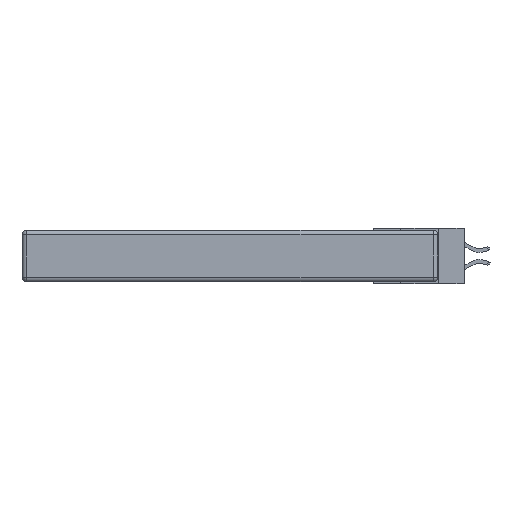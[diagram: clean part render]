
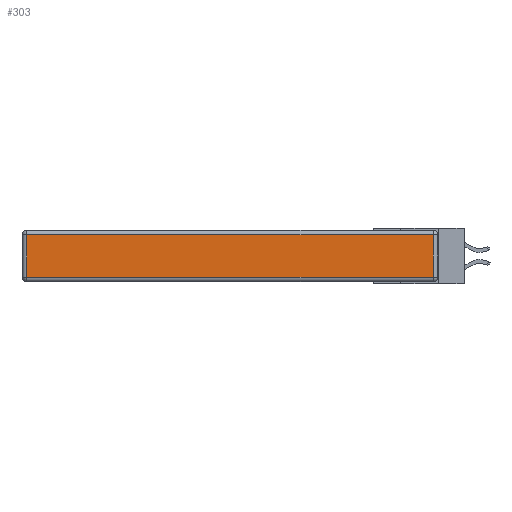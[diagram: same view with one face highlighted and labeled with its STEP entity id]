
A CAD part, left-side view. The second image highlights one B-rep face of the part: STEP entity #303.
In plain terms, the highlighted planar face has unit normal (-1, 0, 0).
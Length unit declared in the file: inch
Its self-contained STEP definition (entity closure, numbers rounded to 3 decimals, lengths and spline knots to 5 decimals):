
#303 = ADVANCED_FACE ( 'NONE', ( #32228 ), #24733, .T. ) ;
#444 = LINE ( 'NONE', #14766, #33903 ) ;
#555 = EDGE_CURVE ( 'NONE', #18209, #25217, #444, .T. ) ;
#1775 = LINE ( 'NONE', #7601, #5133 ) ;
#4228 = CARTESIAN_POINT ( 'NONE',  ( 0., 0.03, -0.313 ) ) ;
#4639 = DIRECTION ( 'NONE',  ( 0., 0., 1. ) ) ;
#4929 = EDGE_CURVE ( 'NONE', #32527, #31891, #1775, .T. ) ;
#5133 = VECTOR ( 'NONE', #13133, 39.37008 ) ;
#6080 = ORIENTED_EDGE ( 'NONE', *, *, #4929, .T. ) ;
#6435 = DIRECTION ( 'NONE',  ( 0., -1., 0. ) ) ;
#7320 = VECTOR ( 'NONE', #6435, 39.37008 ) ;
#7601 = CARTESIAN_POINT ( 'NONE',  ( 0., 2.72, -0.343 ) ) ;
#9018 = LINE ( 'NONE', #20111, #7320 ) ;
#9685 = CARTESIAN_POINT ( 'NONE',  ( 0., 2.75, -0.03 ) ) ;
#13133 = DIRECTION ( 'NONE',  ( 0., 0., -1. ) ) ;
#14091 = DIRECTION ( 'NONE',  ( -1., 0., 0. ) ) ;
#14766 = CARTESIAN_POINT ( 'NONE',  ( 0., 0.03, -0.343 ) ) ;
#14918 = EDGE_CURVE ( 'NONE', #25217, #32527, #32747, .T. ) ;
#16118 = CARTESIAN_POINT ( 'NONE',  ( 0., 2.72, -0.03 ) ) ;
#18209 = VERTEX_POINT ( 'NONE', #4228 ) ;
#20111 = CARTESIAN_POINT ( 'NONE',  ( 0., 0., -0.313 ) ) ;
#22904 = DIRECTION ( 'NONE',  ( 0., 1., 0. ) ) ;
#24622 = CARTESIAN_POINT ( 'NONE',  ( 0., 0., -0.343 ) ) ;
#24733 = PLANE ( 'NONE',  #28168 ) ;
#25217 = VERTEX_POINT ( 'NONE', #26202 ) ;
#25333 = EDGE_LOOP ( 'NONE', ( #29950, #34676, #29292, #6080 ) ) ;
#26202 = CARTESIAN_POINT ( 'NONE',  ( 0., 0.03, -0.03 ) ) ;
#26808 = VECTOR ( 'NONE', #22904, 39.37008 ) ;
#26842 = CARTESIAN_POINT ( 'NONE',  ( 0., 2.72, -0.313 ) ) ;
#27247 = DIRECTION ( 'NONE',  ( 0., 0., 1. ) ) ;
#27876 = EDGE_CURVE ( 'NONE', #31891, #18209, #9018, .T. ) ;
#28168 = AXIS2_PLACEMENT_3D ( 'NONE', #24622, #14091, #27247 ) ;
#29292 = ORIENTED_EDGE ( 'NONE', *, *, #14918, .T. ) ;
#29950 = ORIENTED_EDGE ( 'NONE', *, *, #27876, .T. ) ;
#31891 = VERTEX_POINT ( 'NONE', #26842 ) ;
#32228 = FACE_OUTER_BOUND ( 'NONE', #25333, .T. ) ;
#32527 = VERTEX_POINT ( 'NONE', #16118 ) ;
#32747 = LINE ( 'NONE', #9685, #26808 ) ;
#33903 = VECTOR ( 'NONE', #4639, 39.37008 ) ;
#34676 = ORIENTED_EDGE ( 'NONE', *, *, #555, .T. ) ;
